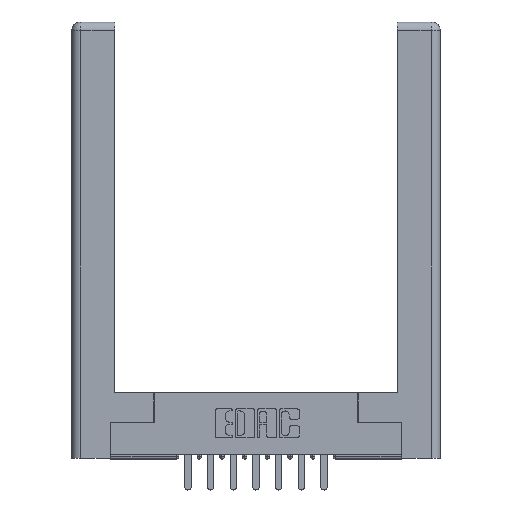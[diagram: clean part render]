
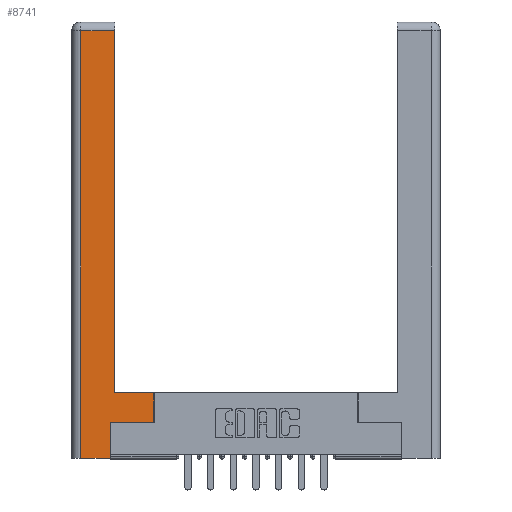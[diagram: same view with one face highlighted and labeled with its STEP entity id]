
A CAD part, top view. The second image highlights one B-rep face of the part: STEP entity #8741.
In plain terms, the highlighted planar face has unit normal (0, 0, 1).
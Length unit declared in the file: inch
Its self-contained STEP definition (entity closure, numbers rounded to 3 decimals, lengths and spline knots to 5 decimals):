
#10 = FACE_OUTER_BOUND ( 'NONE', #3335, .T. ) ;
#327 = ORIENTED_EDGE ( 'NONE', *, *, #9937, .T. ) ;
#738 = LINE ( 'NONE', #2537, #4347 ) ;
#882 = ORIENTED_EDGE ( 'NONE', *, *, #4959, .T. ) ;
#959 = VERTEX_POINT ( 'NONE', #10391 ) ;
#966 = CARTESIAN_POINT ( 'NONE',  ( 0.265, 0., 0. ) ) ;
#1227 = EDGE_CURVE ( 'NONE', #5386, #5326, #7726, .T. ) ;
#1555 = VERTEX_POINT ( 'NONE', #3805 ) ;
#1691 = EDGE_CURVE ( 'NONE', #1555, #5753, #4053, .T. ) ;
#2104 = VECTOR ( 'NONE', #4493, 39.37008 ) ;
#2162 = ORIENTED_EDGE ( 'NONE', *, *, #1227, .T. ) ;
#2313 = VECTOR ( 'NONE', #6045, 39.37008 ) ;
#2537 = CARTESIAN_POINT ( 'NONE',  ( 0.565, 0.45, 0. ) ) ;
#2955 = VECTOR ( 'NONE', #10723, 39.37008 ) ;
#3335 = EDGE_LOOP ( 'NONE', ( #4749, #9727, #2162, #327, #882, #11743, #7536, #5778 ) ) ;
#3629 = CARTESIAN_POINT ( 'NONE',  ( 0.565, 0.45, 0. ) ) ;
#3805 = CARTESIAN_POINT ( 'NONE',  ( 0.295, 0.45, 0. ) ) ;
#3811 = CARTESIAN_POINT ( 'NONE',  ( 0.295, 0.45, 0. ) ) ;
#4053 = LINE ( 'NONE', #8422, #2313 ) ;
#4339 = EDGE_CURVE ( 'NONE', #5753, #5386, #4943, .T. ) ;
#4347 = VECTOR ( 'NONE', #13588, 39.37008 ) ;
#4493 = DIRECTION ( 'NONE',  ( 1., 0., 0. ) ) ;
#4697 = VECTOR ( 'NONE', #8279, 39.37008 ) ;
#4749 = ORIENTED_EDGE ( 'NONE', *, *, #1691, .T. ) ;
#4943 = LINE ( 'NONE', #5246, #12262 ) ;
#4944 = VERTEX_POINT ( 'NONE', #5075 ) ;
#4959 = EDGE_CURVE ( 'NONE', #959, #4944, #8076, .T. ) ;
#5075 = CARTESIAN_POINT ( 'NONE',  ( 0.265, 0.245, 0. ) ) ;
#5246 = CARTESIAN_POINT ( 'NONE',  ( 0.0615, 2.94, 0. ) ) ;
#5285 = DIRECTION ( 'NONE',  ( 0., -1., 0. ) ) ;
#5326 = VERTEX_POINT ( 'NONE', #6926 ) ;
#5386 = VERTEX_POINT ( 'NONE', #5639 ) ;
#5639 = CARTESIAN_POINT ( 'NONE',  ( 0.0615, 2.94, 0. ) ) ;
#5753 = VERTEX_POINT ( 'NONE', #7402 ) ;
#5778 = ORIENTED_EDGE ( 'NONE', *, *, #6740, .T. ) ;
#5783 = CARTESIAN_POINT ( 'NONE',  ( 0.565, 0.245, 0. ) ) ;
#6045 = DIRECTION ( 'NONE',  ( 0., 1., 0. ) ) ;
#6103 = LINE ( 'NONE', #8973, #2104 ) ;
#6740 = EDGE_CURVE ( 'NONE', #7935, #1555, #13782, .T. ) ;
#6926 = CARTESIAN_POINT ( 'NONE',  ( 0.0615, 0., 0. ) ) ;
#7024 = VECTOR ( 'NONE', #7317, 39.37008 ) ;
#7268 = DIRECTION ( 'NONE',  ( 0., 0., -1. ) ) ;
#7317 = DIRECTION ( 'NONE',  ( 0., 1., 0. ) ) ;
#7402 = CARTESIAN_POINT ( 'NONE',  ( 0.295, 2.94, 0. ) ) ;
#7536 = ORIENTED_EDGE ( 'NONE', *, *, #12141, .T. ) ;
#7726 = LINE ( 'NONE', #11950, #10484 ) ;
#7935 = VERTEX_POINT ( 'NONE', #3629 ) ;
#8040 = CARTESIAN_POINT ( 'NONE',  ( 0.265, 0.245, 0. ) ) ;
#8076 = LINE ( 'NONE', #8040, #7024 ) ;
#8279 = DIRECTION ( 'NONE',  ( -1., 0., 0. ) ) ;
#8422 = CARTESIAN_POINT ( 'NONE',  ( 0.295, 3., 0. ) ) ;
#8741 = ADVANCED_FACE ( 'NONE', ( #10 ), #12920, .F. ) ;
#8973 = CARTESIAN_POINT ( 'NONE',  ( 0.565, 0.245, 0. ) ) ;
#9727 = ORIENTED_EDGE ( 'NONE', *, *, #4339, .T. ) ;
#9937 = EDGE_CURVE ( 'NONE', #5326, #959, #12501, .T. ) ;
#10391 = CARTESIAN_POINT ( 'NONE',  ( 0.265, 0., 0. ) ) ;
#10484 = VECTOR ( 'NONE', #5285, 39.37008 ) ;
#10723 = DIRECTION ( 'NONE',  ( 1., 0., 0. ) ) ;
#10732 = DIRECTION ( 'NONE',  ( -1., 0., 0. ) ) ;
#11249 = EDGE_CURVE ( 'NONE', #4944, #13271, #6103, .T. ) ;
#11743 = ORIENTED_EDGE ( 'NONE', *, *, #11249, .T. ) ;
#11925 = DIRECTION ( 'NONE',  ( -1., 0., 0. ) ) ;
#11950 = CARTESIAN_POINT ( 'NONE',  ( 0.0615, 0., 0. ) ) ;
#12141 = EDGE_CURVE ( 'NONE', #13271, #7935, #738, .T. ) ;
#12262 = VECTOR ( 'NONE', #10732, 39.37008 ) ;
#12501 = LINE ( 'NONE', #966, #2955 ) ;
#12620 = AXIS2_PLACEMENT_3D ( 'NONE', #14093, #7268, #11925 ) ;
#12920 = PLANE ( 'NONE',  #12620 ) ;
#13271 = VERTEX_POINT ( 'NONE', #5783 ) ;
#13588 = DIRECTION ( 'NONE',  ( 0., 1., 0. ) ) ;
#13782 = LINE ( 'NONE', #3811, #4697 ) ;
#14093 = CARTESIAN_POINT ( 'NONE',  ( 0., 0., 0. ) ) ;
